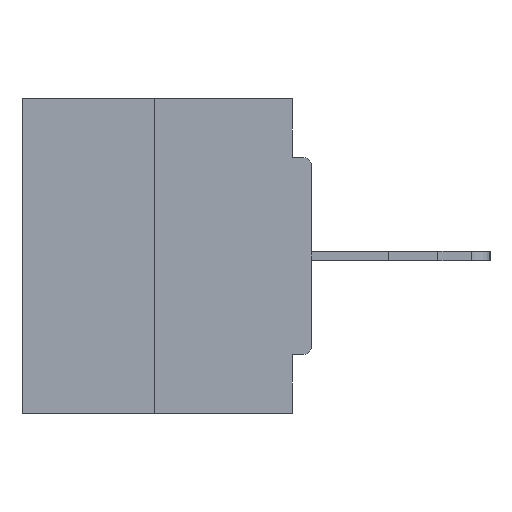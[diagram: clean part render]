
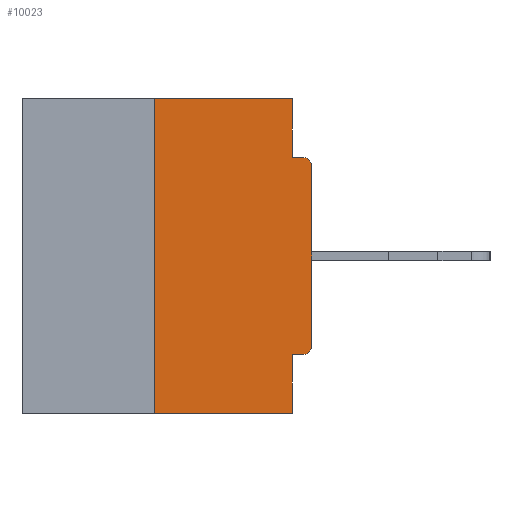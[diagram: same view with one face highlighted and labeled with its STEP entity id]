
A CAD part, left-side view. The second image highlights one B-rep face of the part: STEP entity #10023.
In plain terms, the highlighted planar face has unit normal (-1, 0, 0).
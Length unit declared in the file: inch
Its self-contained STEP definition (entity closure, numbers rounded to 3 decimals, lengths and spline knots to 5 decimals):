
#122 = LINE ( 'NONE', #13402, #6729 ) ;
#550 = ORIENTED_EDGE ( 'NONE', *, *, #2695, .F. ) ;
#554 = FACE_OUTER_BOUND ( 'NONE', #3689, .T. ) ;
#1050 = ORIENTED_EDGE ( 'NONE', *, *, #6024, .T. ) ;
#1787 = CARTESIAN_POINT ( 'NONE',  ( 0., 0.031, 0. ) ) ;
#2093 = CARTESIAN_POINT ( 'NONE',  ( 0., 0., -0.0935 ) ) ;
#2234 = LINE ( 'NONE', #2093, #13925 ) ;
#2353 = DIRECTION ( 'NONE',  ( -1., 0., 0. ) ) ;
#2683 = VERTEX_POINT ( 'NONE', #27770 ) ;
#2695 = EDGE_CURVE ( 'NONE', #10622, #4552, #2234, .T. ) ;
#2824 = DIRECTION ( 'NONE',  ( -1., 0., 0. ) ) ;
#3689 = EDGE_LOOP ( 'NONE', ( #18497, #4312, #1050, #27005, #21184, #7296, #10193, #13353, #550, #17292 ) ) ;
#3794 = EDGE_CURVE ( 'NONE', #2683, #21385, #20595, .T. ) ;
#3944 = VECTOR ( 'NONE', #25800, 39.37008 ) ;
#4312 = ORIENTED_EDGE ( 'NONE', *, *, #17304, .F. ) ;
#4552 = VERTEX_POINT ( 'NONE', #14315 ) ;
#4693 = VERTEX_POINT ( 'NONE', #14594 ) ;
#4744 = VERTEX_POINT ( 'NONE', #17035 ) ;
#4843 = VECTOR ( 'NONE', #20625, 39.37008 ) ;
#5202 = CARTESIAN_POINT ( 'NONE',  ( 0., 0.031, -0.5 ) ) ;
#5319 = DIRECTION ( 'NONE',  ( 1., 0., 0. ) ) ;
#5576 = CARTESIAN_POINT ( 'NONE',  ( 0., 0.46, -0.5 ) ) ;
#5584 = CARTESIAN_POINT ( 'NONE',  ( 0., 0.46, 0. ) ) ;
#5613 = EDGE_CURVE ( 'NONE', #21385, #10622, #21525, .T. ) ;
#5721 = EDGE_CURVE ( 'NONE', #7903, #4552, #25516, .T. ) ;
#6024 = EDGE_CURVE ( 'NONE', #23750, #8472, #16545, .T. ) ;
#6729 = VECTOR ( 'NONE', #9074, 39.37008 ) ;
#7029 = CIRCLE ( 'NONE', #20834, 0.015 ) ;
#7296 = ORIENTED_EDGE ( 'NONE', *, *, #10412, .T. ) ;
#7788 = EDGE_CURVE ( 'NONE', #4693, #8472, #28157, .T. ) ;
#7903 = VERTEX_POINT ( 'NONE', #24393 ) ;
#8040 = AXIS2_PLACEMENT_3D ( 'NONE', #20248, #2353, #26421 ) ;
#8096 = CARTESIAN_POINT ( 'NONE',  ( 0., 0.25, 0. ) ) ;
#8472 = VERTEX_POINT ( 'NONE', #5202 ) ;
#8860 = DIRECTION ( 'NONE',  ( 0., -1., 0. ) ) ;
#9074 = DIRECTION ( 'NONE',  ( 0., 0., 1. ) ) ;
#9760 = DIRECTION ( 'NONE',  ( 0., -1., 0. ) ) ;
#10023 = ADVANCED_FACE ( 'NONE', ( #554 ), #18570, .F. ) ;
#10193 = ORIENTED_EDGE ( 'NONE', *, *, #27631, .T. ) ;
#10412 = EDGE_CURVE ( 'NONE', #12847, #4744, #7029, .T. ) ;
#10445 = CARTESIAN_POINT ( 'NONE',  ( 0., 0.031, -0.0935 ) ) ;
#10622 = VERTEX_POINT ( 'NONE', #10445 ) ;
#11237 = CARTESIAN_POINT ( 'NONE',  ( 0., 0.015, -0.4065 ) ) ;
#11836 = LINE ( 'NONE', #18027, #4843 ) ;
#12847 = VERTEX_POINT ( 'NONE', #11237 ) ;
#12882 = CARTESIAN_POINT ( 'NONE',  ( 0., 0.031, -0.5 ) ) ;
#13353 = ORIENTED_EDGE ( 'NONE', *, *, #5721, .T. ) ;
#13402 = CARTESIAN_POINT ( 'NONE',  ( 0., 0., 0. ) ) ;
#13925 = VECTOR ( 'NONE', #8860, 39.37008 ) ;
#13929 = AXIS2_PLACEMENT_3D ( 'NONE', #25051, #5319, #24775 ) ;
#14315 = CARTESIAN_POINT ( 'NONE',  ( 0., 0.015, -0.0935 ) ) ;
#14594 = CARTESIAN_POINT ( 'NONE',  ( 0., 0.031, -0.4065 ) ) ;
#15899 = VECTOR ( 'NONE', #19655, 39.37008 ) ;
#15962 = CARTESIAN_POINT ( 'NONE',  ( 0., 0.015, -0.3915 ) ) ;
#16366 = EDGE_CURVE ( 'NONE', #12847, #4693, #11836, .T. ) ;
#16545 = LINE ( 'NONE', #5576, #28283 ) ;
#17035 = CARTESIAN_POINT ( 'NONE',  ( 0., 0., -0.3915 ) ) ;
#17292 = ORIENTED_EDGE ( 'NONE', *, *, #5613, .F. ) ;
#17304 = EDGE_CURVE ( 'NONE', #23750, #2683, #23229, .T. ) ;
#18027 = CARTESIAN_POINT ( 'NONE',  ( 0., 0., -0.4065 ) ) ;
#18263 = CARTESIAN_POINT ( 'NONE',  ( 0., 0.031, 0. ) ) ;
#18497 = ORIENTED_EDGE ( 'NONE', *, *, #3794, .F. ) ;
#18570 = PLANE ( 'NONE',  #13929 ) ;
#18951 = CARTESIAN_POINT ( 'NONE',  ( 0., 0.25, -0.5 ) ) ;
#18976 = DIRECTION ( 'NONE',  ( 0., -1., 0. ) ) ;
#19655 = DIRECTION ( 'NONE',  ( 0., 0., -1. ) ) ;
#20248 = CARTESIAN_POINT ( 'NONE',  ( 0., 0.015, -0.1085 ) ) ;
#20569 = DIRECTION ( 'NONE',  ( 0., 0., -1. ) ) ;
#20595 = LINE ( 'NONE', #5584, #21741 ) ;
#20625 = DIRECTION ( 'NONE',  ( 0., 1., 0. ) ) ;
#20834 = AXIS2_PLACEMENT_3D ( 'NONE', #15962, #2824, #20569 ) ;
#21184 = ORIENTED_EDGE ( 'NONE', *, *, #16366, .F. ) ;
#21385 = VERTEX_POINT ( 'NONE', #18263 ) ;
#21525 = LINE ( 'NONE', #1787, #22776 ) ;
#21741 = VECTOR ( 'NONE', #18976, 39.37008 ) ;
#22776 = VECTOR ( 'NONE', #27898, 39.37008 ) ;
#23229 = LINE ( 'NONE', #8096, #3944 ) ;
#23750 = VERTEX_POINT ( 'NONE', #18951 ) ;
#24393 = CARTESIAN_POINT ( 'NONE',  ( 0., 0., -0.1085 ) ) ;
#24775 = DIRECTION ( 'NONE',  ( 0., 0., -1. ) ) ;
#25051 = CARTESIAN_POINT ( 'NONE',  ( 0., 0.46, 0. ) ) ;
#25516 = CIRCLE ( 'NONE', #8040, 0.015 ) ;
#25800 = DIRECTION ( 'NONE',  ( 0., 0., 1. ) ) ;
#26421 = DIRECTION ( 'NONE',  ( 0., 0., -1. ) ) ;
#27005 = ORIENTED_EDGE ( 'NONE', *, *, #7788, .F. ) ;
#27631 = EDGE_CURVE ( 'NONE', #4744, #7903, #122, .T. ) ;
#27770 = CARTESIAN_POINT ( 'NONE',  ( 0., 0.25, 0. ) ) ;
#27898 = DIRECTION ( 'NONE',  ( 0., 0., -1. ) ) ;
#28157 = LINE ( 'NONE', #12882, #15899 ) ;
#28283 = VECTOR ( 'NONE', #9760, 39.37008 ) ;
